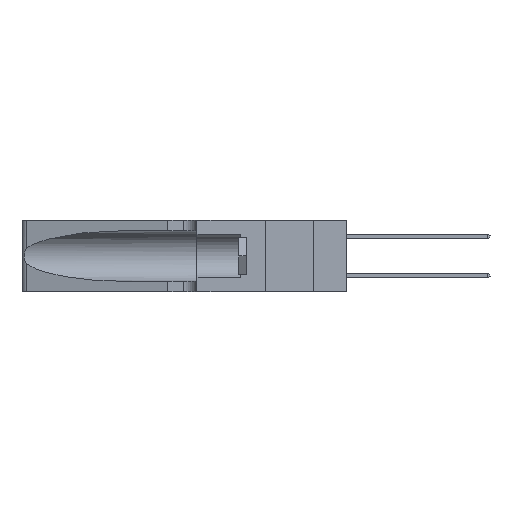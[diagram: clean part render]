
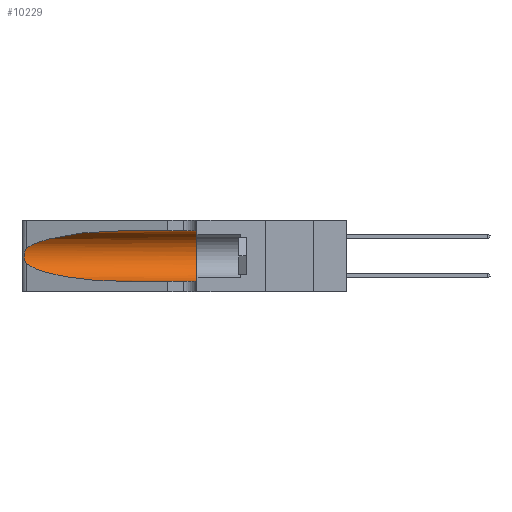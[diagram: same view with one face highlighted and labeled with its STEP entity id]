
A CAD part, left-side view. The second image highlights one B-rep face of the part: STEP entity #10229.
In plain terms, the highlighted cylindrical face has radius 3.308 mm (diameter 6.617 mm), a partial arc.
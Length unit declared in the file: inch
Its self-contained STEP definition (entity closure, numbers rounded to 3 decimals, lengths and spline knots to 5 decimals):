
#1543 = VERTEX_POINT ( 'NONE', #28216 ) ;
#5229 =( BOUNDED_CURVE ( )  B_SPLINE_CURVE ( 3, ( #12078, #34576, #19669, #45864 ),
 .UNSPECIFIED., .F., .T. ) 
 B_SPLINE_CURVE_WITH_KNOTS ( ( 4, 4 ),
 ( 1.5708, 2.84003 ),
 .UNSPECIFIED. ) 
 CURVE ( )  GEOMETRIC_REPRESENTATION_ITEM ( )  RATIONAL_B_SPLINE_CURVE ( ( 1., 0.87, 0.87, 1. ) ) 
 REPRESENTATION_ITEM ( '' )  );
#5557 = CARTESIAN_POINT ( 'NONE',  ( 0.1305, 0.72297, 0.31525 ) ) ;
#7032 = CARTESIAN_POINT ( 'NONE',  ( 0.25787, 1.23484, 0.2124 ) ) ;
#7608 = CARTESIAN_POINT ( 'NONE',  ( 0.18966, 0.96281, 0.05475 ) ) ;
#8302 = VERTEX_POINT ( 'NONE', #5557 ) ;
#8580 = EDGE_CURVE ( 'NONE', #20319, #23765, #43892, .T. ) ;
#8727 = VECTOR ( 'NONE', #43992, 39.37008 ) ;
#10158 = DIRECTION ( 'NONE',  ( 0., 1., 0. ) ) ;
#10229 = ADVANCED_FACE ( 'NONE', ( #35854 ), #44637, .F. ) ;
#10902 = CARTESIAN_POINT ( 'NONE',  ( 0.26018, 1.23835, 0.19895 ) ) ;
#11259 = VERTEX_POINT ( 'NONE', #12023 ) ;
#12023 = CARTESIAN_POINT ( 'NONE',  ( 0.1305, 0.35, 0.31525 ) ) ;
#12078 = CARTESIAN_POINT ( 'NONE',  ( 0.1305, 0.72297, 0.31525 ) ) ;
#13075 = CARTESIAN_POINT ( 'NONE',  ( 0.1305, 0.35, 0.05475 ) ) ;
#14710 = CARTESIAN_POINT ( 'NONE',  ( 0.26075, 1.23896, 0.178 ) ) ;
#18487 = CARTESIAN_POINT ( 'NONE',  ( 0.25856, 1.23593, 0.16098 ) ) ;
#19407 = CARTESIAN_POINT ( 'NONE',  ( 0.1305, 1.61858, 0.05475 ) ) ;
#19645 = CIRCLE ( 'NONE', #41417, 0.13025 ) ;
#19669 = CARTESIAN_POINT ( 'NONE',  ( 0.2373, 1.15595, 0.28018 ) ) ;
#20319 = VERTEX_POINT ( 'NONE', #32218 ) ;
#20927 = VECTOR ( 'NONE', #30752, 39.37008 ) ;
#21564 = DIRECTION ( 'NONE',  ( 0., -1., 0. ) ) ;
#21600 = CARTESIAN_POINT ( 'NONE',  ( 0.1305, 1.61858, 0.31525 ) ) ;
#21864 = AXIS2_PLACEMENT_3D ( 'NONE', #28937, #21564, #47736 ) ;
#22165 = CARTESIAN_POINT ( 'NONE',  ( 0.25639, 1.23184, 0.21858 ) ) ;
#22322 = CARTESIAN_POINT ( 'NONE',  ( 0.25639, 1.23186, 0.15144 ) ) ;
#23765 = VERTEX_POINT ( 'NONE', #42173 ) ;
#23838 = EDGE_LOOP ( 'NONE', ( #42071, #43271, #34468, #26900, #46788, #28079 ) ) ;
#26090 = CARTESIAN_POINT ( 'NONE',  ( 0.25487, 1.22718, 0.14631 ) ) ;
#26505 = CARTESIAN_POINT ( 'NONE',  ( 0.25487, 1.22718, 0.14631 ) ) ;
#26900 = ORIENTED_EDGE ( 'NONE', *, *, #40169, .T. ) ;
#28079 = ORIENTED_EDGE ( 'NONE', *, *, #35071, .F. ) ;
#28216 = CARTESIAN_POINT ( 'NONE',  ( 0.1305, 0.72297, 0.05475 ) ) ;
#28937 = CARTESIAN_POINT ( 'NONE',  ( 0.1305, 1.61858, 0.185 ) ) ;
#29708 = CARTESIAN_POINT ( 'NONE',  ( 0.25487, 1.22718, 0.22369 ) ) ;
#30270 = CARTESIAN_POINT ( 'NONE',  ( 0.2373, 1.15595, 0.08982 ) ) ;
#30752 = DIRECTION ( 'NONE',  ( 0., -1., 0. ) ) ;
#31623 =( BOUNDED_CURVE ( )  B_SPLINE_CURVE ( 3, ( #26505, #30270, #7608, #33995 ),
 .UNSPECIFIED., .F., .T. ) 
 B_SPLINE_CURVE_WITH_KNOTS ( ( 4, 4 ),
 ( 3.44316, 4.71239 ),
 .UNSPECIFIED. ) 
 CURVE ( )  GEOMETRIC_REPRESENTATION_ITEM ( )  RATIONAL_B_SPLINE_CURVE ( ( 1., 0.87, 0.87, 1. ) ) 
 REPRESENTATION_ITEM ( '' )  );
#32084 = LINE ( 'NONE', #19407, #20927 ) ;
#32218 = CARTESIAN_POINT ( 'NONE',  ( 0.25487, 1.22718, 0.22369 ) ) ;
#32320 = EDGE_CURVE ( 'NONE', #23765, #1543, #31623, .T. ) ;
#32738 = CARTESIAN_POINT ( 'NONE',  ( 0.1305, 0.35, 0.185 ) ) ;
#33444 = CARTESIAN_POINT ( 'NONE',  ( 0.25854, 1.2359, 0.20912 ) ) ;
#33995 = CARTESIAN_POINT ( 'NONE',  ( 0.1305, 0.72297, 0.05475 ) ) ;
#34177 = VERTEX_POINT ( 'NONE', #13075 ) ;
#34468 = ORIENTED_EDGE ( 'NONE', *, *, #32320, .T. ) ;
#34576 = CARTESIAN_POINT ( 'NONE',  ( 0.18966, 0.96281, 0.31525 ) ) ;
#35071 = EDGE_CURVE ( 'NONE', #8302, #11259, #46389, .T. ) ;
#35854 = FACE_OUTER_BOUND ( 'NONE', #23838, .T. ) ;
#35918 = EDGE_CURVE ( 'NONE', #8302, #20319, #5229, .T. ) ;
#36484 = DIRECTION ( 'NONE',  ( 0., 0., 1. ) ) ;
#37034 = CARTESIAN_POINT ( 'NONE',  ( 0.25555, 1.22994, 0.2215 ) ) ;
#37203 = CARTESIAN_POINT ( 'NONE',  ( 0.26075, 1.23896, 0.19203 ) ) ;
#38550 = EDGE_CURVE ( 'NONE', #11259, #34177, #19645, .T. ) ;
#40169 = EDGE_CURVE ( 'NONE', #1543, #34177, #32084, .T. ) ;
#40955 = CARTESIAN_POINT ( 'NONE',  ( 0.26017, 1.23833, 0.17102 ) ) ;
#41417 = AXIS2_PLACEMENT_3D ( 'NONE', #32738, #10158, #36484 ) ;
#42071 = ORIENTED_EDGE ( 'NONE', *, *, #35918, .T. ) ;
#42173 = CARTESIAN_POINT ( 'NONE',  ( 0.25487, 1.22718, 0.14631 ) ) ;
#43271 = ORIENTED_EDGE ( 'NONE', *, *, #8580, .T. ) ;
#43892 = B_SPLINE_CURVE_WITH_KNOTS ( 'NONE', 3,
 ( #29708, #37034, #22165, #7032, #33444, #10902, #37203, #14710, #40955, #18487, #44712, #22322, #48491, #26090 ),
 .UNSPECIFIED., .F., .F.,
 ( 4, 2, 2, 2, 2, 2, 4 ),
 ( 0., 0.00027, 0.00053, 0.00107, 0.0016, 0.00187, 0.00214 ),
 .UNSPECIFIED. ) ;
#43992 = DIRECTION ( 'NONE',  ( 0., -1., 0. ) ) ;
#44637 = CYLINDRICAL_SURFACE ( 'NONE', #21864, 0.13025 ) ;
#44712 = CARTESIAN_POINT ( 'NONE',  ( 0.25789, 1.23486, 0.15765 ) ) ;
#45864 = CARTESIAN_POINT ( 'NONE',  ( 0.25487, 1.22718, 0.22369 ) ) ;
#46389 = LINE ( 'NONE', #21600, #8727 ) ;
#46788 = ORIENTED_EDGE ( 'NONE', *, *, #38550, .F. ) ;
#47736 = DIRECTION ( 'NONE',  ( 0., 0., -1. ) ) ;
#48491 = CARTESIAN_POINT ( 'NONE',  ( 0.25555, 1.22993, 0.14849 ) ) ;
